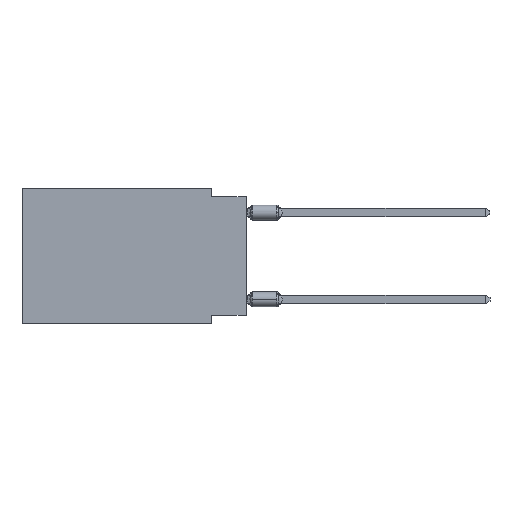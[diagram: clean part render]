
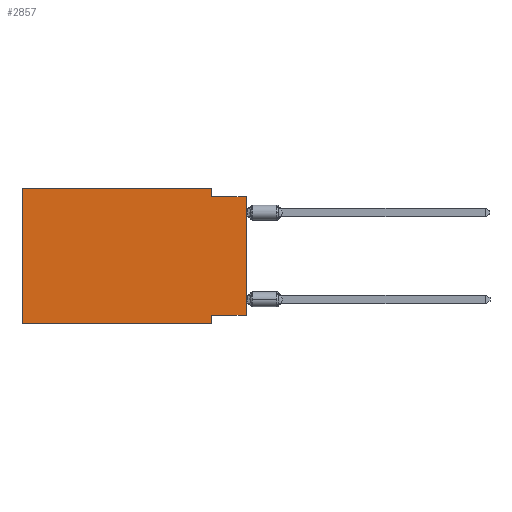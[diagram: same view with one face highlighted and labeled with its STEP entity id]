
A CAD part, left-side view. The second image highlights one B-rep face of the part: STEP entity #2857.
In plain terms, the highlighted planar face has unit normal (-1, 0, 0).
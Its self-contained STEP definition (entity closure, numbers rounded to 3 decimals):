
#4 = CARTESIAN_POINT ( 'NONE',  ( 0., 2.54, -9.906 ) ) ;
#403 = DIRECTION ( 'NONE',  ( 0., 1., 0. ) ) ;
#786 = ORIENTED_EDGE ( 'NONE', *, *, #14955, .F. ) ;
#810 = VECTOR ( 'NONE', #9510, 1000. ) ;
#1398 = CARTESIAN_POINT ( 'NONE',  ( 0., 0., -9.271 ) ) ;
#1773 = VERTEX_POINT ( 'NONE', #13877 ) ;
#2010 = LINE ( 'NONE', #7896, #3038 ) ;
#2087 = CARTESIAN_POINT ( 'NONE',  ( 0., 16.383, -9.906 ) ) ;
#2193 = VERTEX_POINT ( 'NONE', #8976 ) ;
#2552 = EDGE_CURVE ( 'NONE', #13795, #2924, #11424, .T. ) ;
#2857 = ADVANCED_FACE ( 'NONE', ( #7340 ), #11016, .F. ) ;
#2924 = VERTEX_POINT ( 'NONE', #14455 ) ;
#2955 = EDGE_CURVE ( 'NONE', #1773, #4643, #6073, .T. ) ;
#3038 = VECTOR ( 'NONE', #12946, 1000. ) ;
#3040 = CARTESIAN_POINT ( 'NONE',  ( 0., 16.383, -9.906 ) ) ;
#3998 = CARTESIAN_POINT ( 'NONE',  ( 0., 0., -9.271 ) ) ;
#4411 = LINE ( 'NONE', #7824, #13301 ) ;
#4642 = CARTESIAN_POINT ( 'NONE',  ( 0., 0., 0. ) ) ;
#4643 = VERTEX_POINT ( 'NONE', #9566 ) ;
#4848 = VECTOR ( 'NONE', #403, 1000. ) ;
#4873 = DIRECTION ( 'NONE',  ( 0., 0., -1. ) ) ;
#4959 = DIRECTION ( 'NONE',  ( 0., 0., -1. ) ) ;
#5141 = VECTOR ( 'NONE', #4873, 1000. ) ;
#5219 = ORIENTED_EDGE ( 'NONE', *, *, #6856, .F. ) ;
#5513 = ORIENTED_EDGE ( 'NONE', *, *, #2955, .F. ) ;
#5564 = VERTEX_POINT ( 'NONE', #1398 ) ;
#5681 = LINE ( 'NONE', #3040, #7123 ) ;
#5932 = EDGE_LOOP ( 'NONE', ( #7904, #11029, #11062, #6473, #786, #12889, #5513, #5219 ) ) ;
#6073 = LINE ( 'NONE', #4, #5141 ) ;
#6162 = VECTOR ( 'NONE', #9916, 1000. ) ;
#6473 = ORIENTED_EDGE ( 'NONE', *, *, #14879, .F. ) ;
#6856 = EDGE_CURVE ( 'NONE', #5564, #1773, #10288, .T. ) ;
#7123 = VECTOR ( 'NONE', #7891, 1000. ) ;
#7340 = FACE_OUTER_BOUND ( 'NONE', #5932, .T. ) ;
#7666 = CARTESIAN_POINT ( 'NONE',  ( 0., 2.54, 0. ) ) ;
#7824 = CARTESIAN_POINT ( 'NONE',  ( 0., 0., -0.635 ) ) ;
#7891 = DIRECTION ( 'NONE',  ( 0., -1., 0. ) ) ;
#7896 = CARTESIAN_POINT ( 'NONE',  ( 0., 16.383, 0. ) ) ;
#7904 = ORIENTED_EDGE ( 'NONE', *, *, #8391, .T. ) ;
#8094 = CARTESIAN_POINT ( 'NONE',  ( 0., 2.54, 0. ) ) ;
#8186 = EDGE_CURVE ( 'NONE', #2924, #2193, #4411, .T. ) ;
#8368 = DIRECTION ( 'NONE',  ( 0., 0., 1. ) ) ;
#8391 = EDGE_CURVE ( 'NONE', #5564, #2193, #9586, .T. ) ;
#8976 = CARTESIAN_POINT ( 'NONE',  ( 0., 0., -0.635 ) ) ;
#9025 = VERTEX_POINT ( 'NONE', #9601 ) ;
#9510 = DIRECTION ( 'NONE',  ( 0., 0., 1. ) ) ;
#9566 = CARTESIAN_POINT ( 'NONE',  ( 0., 2.54, -9.906 ) ) ;
#9586 = LINE ( 'NONE', #4642, #810 ) ;
#9601 = CARTESIAN_POINT ( 'NONE',  ( 0., 16.383, 0. ) ) ;
#9916 = DIRECTION ( 'NONE',  ( 0., 0., -1. ) ) ;
#10162 = VECTOR ( 'NONE', #8368, 1000. ) ;
#10288 = LINE ( 'NONE', #3998, #4848 ) ;
#10742 = EDGE_CURVE ( 'NONE', #11832, #4643, #5681, .T. ) ;
#10784 = CARTESIAN_POINT ( 'NONE',  ( 0., 16.383, 0. ) ) ;
#11016 = PLANE ( 'NONE',  #14583 ) ;
#11029 = ORIENTED_EDGE ( 'NONE', *, *, #8186, .F. ) ;
#11062 = ORIENTED_EDGE ( 'NONE', *, *, #2552, .F. ) ;
#11424 = LINE ( 'NONE', #7666, #6162 ) ;
#11832 = VERTEX_POINT ( 'NONE', #2087 ) ;
#12709 = DIRECTION ( 'NONE',  ( 0., -1., 0. ) ) ;
#12889 = ORIENTED_EDGE ( 'NONE', *, *, #10742, .T. ) ;
#12946 = DIRECTION ( 'NONE',  ( 0., -1., 0. ) ) ;
#13301 = VECTOR ( 'NONE', #12709, 1000. ) ;
#13333 = CARTESIAN_POINT ( 'NONE',  ( 0., 16.383, 0. ) ) ;
#13795 = VERTEX_POINT ( 'NONE', #8094 ) ;
#13877 = CARTESIAN_POINT ( 'NONE',  ( 0., 2.54, -9.271 ) ) ;
#14385 = DIRECTION ( 'NONE',  ( 1., 0., 0. ) ) ;
#14455 = CARTESIAN_POINT ( 'NONE',  ( 0., 2.54, -0.635 ) ) ;
#14583 = AXIS2_PLACEMENT_3D ( 'NONE', #10784, #14385, #4959 ) ;
#14879 = EDGE_CURVE ( 'NONE', #9025, #13795, #2010, .T. ) ;
#14955 = EDGE_CURVE ( 'NONE', #11832, #9025, #15475, .T. ) ;
#15475 = LINE ( 'NONE', #13333, #10162 ) ;
